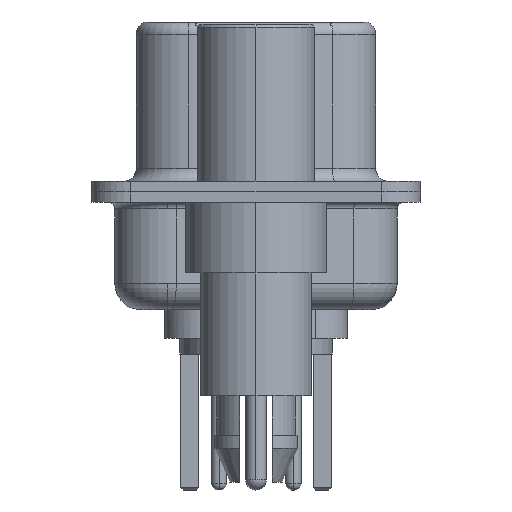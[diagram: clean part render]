
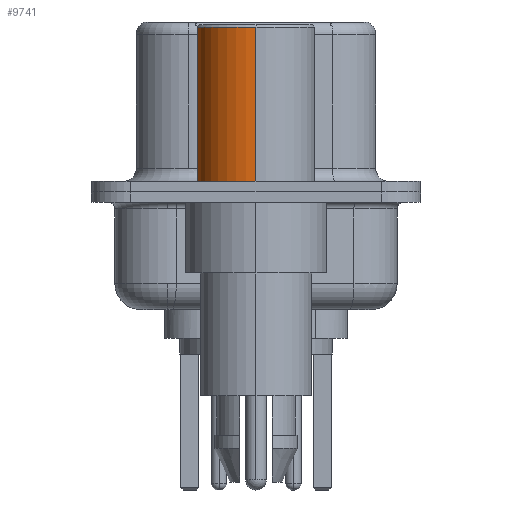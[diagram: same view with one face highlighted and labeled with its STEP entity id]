
A CAD part, left-side view. The second image highlights one B-rep face of the part: STEP entity #9741.
In plain terms, the highlighted cylindrical face has radius 2.25 mm (diameter 4.5 mm), a partial arc.
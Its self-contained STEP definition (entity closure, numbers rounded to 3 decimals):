
#289 = VERTEX_POINT ( 'NONE', #8190 ) ;
#406 = FACE_OUTER_BOUND ( 'NONE', #11031, .T. ) ;
#1080 = CARTESIAN_POINT ( 'NONE',  ( 0., 0., 0.4 ) ) ;
#2794 = DIRECTION ( 'NONE',  ( 1., 0., 0. ) ) ;
#3436 = ORIENTED_EDGE ( 'NONE', *, *, #14952, .F. ) ;
#4172 = CIRCLE ( 'NONE', #10598, 2.25 ) ;
#4735 = CARTESIAN_POINT ( 'NONE',  ( 2.25, 0., 0.581 ) ) ;
#5064 = EDGE_CURVE ( 'NONE', #18852, #18066, #5111, .T. ) ;
#5111 = LINE ( 'NONE', #20616, #13660 ) ;
#5583 = ORIENTED_EDGE ( 'NONE', *, *, #20052, .T. ) ;
#7897 = CARTESIAN_POINT ( 'NONE',  ( -2.25, 0., 6.3 ) ) ;
#8133 = DIRECTION ( 'NONE',  ( 0., 0., 1. ) ) ;
#8190 = CARTESIAN_POINT ( 'NONE',  ( 2.25, 0., 0.4 ) ) ;
#8646 = DIRECTION ( 'NONE',  ( 0., 0., 1. ) ) ;
#9712 = CARTESIAN_POINT ( 'NONE',  ( 0., 0., 6.3 ) ) ;
#9741 = ADVANCED_FACE ( 'NONE', ( #406 ), #17516, .T. ) ;
#9760 = CARTESIAN_POINT ( 'NONE',  ( 2.25, 0., 6.3 ) ) ;
#9786 = EDGE_CURVE ( 'NONE', #289, #22124, #16978, .T. ) ;
#10598 = AXIS2_PLACEMENT_3D ( 'NONE', #1080, #12996, #2794 ) ;
#11031 = EDGE_LOOP ( 'NONE', ( #5583, #17271, #3436, #18166 ) ) ;
#11387 = DIRECTION ( 'NONE',  ( 0., 0., 1. ) ) ;
#11415 = DIRECTION ( 'NONE',  ( 1., 0., 0. ) ) ;
#11945 = CARTESIAN_POINT ( 'NONE',  ( -2.25, 0., 0.4 ) ) ;
#12996 = DIRECTION ( 'NONE',  ( 0., 0., 1. ) ) ;
#13660 = VECTOR ( 'NONE', #8646, 1000. ) ;
#14952 = EDGE_CURVE ( 'NONE', #22124, #18066, #15230, .T. ) ;
#15230 = CIRCLE ( 'NONE', #18102, 2.25 ) ;
#16559 = CARTESIAN_POINT ( 'NONE',  ( 0., 0., 0.581 ) ) ;
#16978 = LINE ( 'NONE', #4735, #20992 ) ;
#17271 = ORIENTED_EDGE ( 'NONE', *, *, #5064, .T. ) ;
#17516 = CYLINDRICAL_SURFACE ( 'NONE', #17678, 2.25 ) ;
#17678 = AXIS2_PLACEMENT_3D ( 'NONE', #16559, #11387, #20004 ) ;
#18066 = VERTEX_POINT ( 'NONE', #7897 ) ;
#18102 = AXIS2_PLACEMENT_3D ( 'NONE', #9712, #21700, #11415 ) ;
#18166 = ORIENTED_EDGE ( 'NONE', *, *, #9786, .F. ) ;
#18852 = VERTEX_POINT ( 'NONE', #11945 ) ;
#20004 = DIRECTION ( 'NONE',  ( 1., 0., 0. ) ) ;
#20052 = EDGE_CURVE ( 'NONE', #289, #18852, #4172, .T. ) ;
#20616 = CARTESIAN_POINT ( 'NONE',  ( -2.25, 0., 0.581 ) ) ;
#20992 = VECTOR ( 'NONE', #8133, 1000. ) ;
#21700 = DIRECTION ( 'NONE',  ( 0., 0., 1. ) ) ;
#22124 = VERTEX_POINT ( 'NONE', #9760 ) ;
